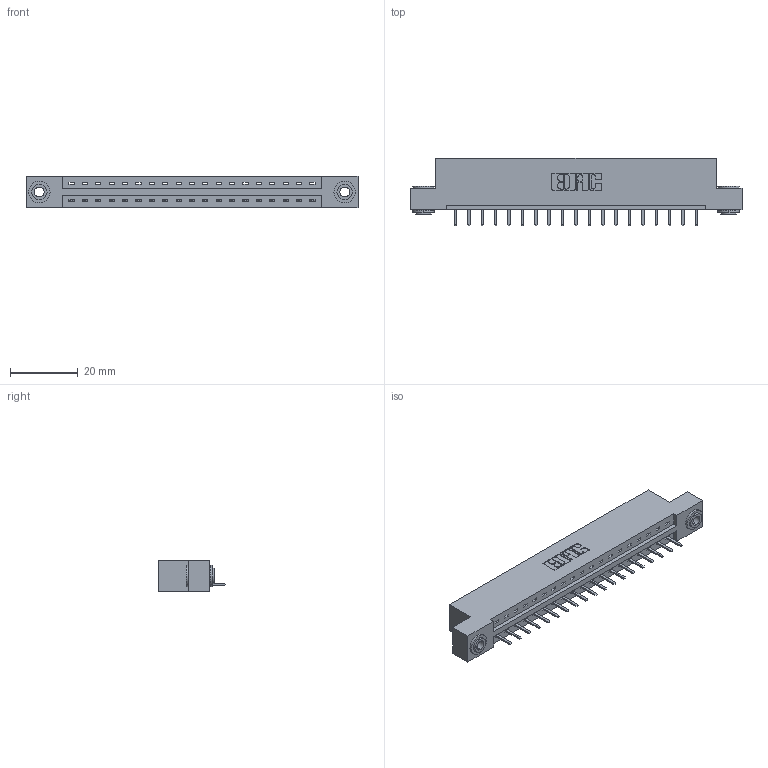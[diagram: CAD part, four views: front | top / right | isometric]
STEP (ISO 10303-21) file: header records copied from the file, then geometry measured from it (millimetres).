
FILE_DESCRIPTION (( 'STEP AP203' ), '1' );
FILE_NAME ('387-019-520-103.STEP', '2019-10-02T20:51:20', ( '' ), ( '' ), 'SwSTEP 2.0', 'SolidWorks 2016', '' );
FILE_SCHEMA (( 'CONFIG_CONTROL_DESIGN' ));
Length unit declared in the file: inch
Products named in the file (4): 337 Part_Flush Mounting Lugs - 0.156 Dia-TH; 387-019-520-103; 345-250-002_345-250-002-102; 345-292-001_345-293-120
Assembly tree (22 placements, depth 2):
  387-019-520-103
    337 Part_Flush Mounting Lugs - 0.156 Dia-TH
    345-292-001_345-293-120  x19
    345-250-002_345-250-002-102  x2
Bounding box: 98.3 x 20.02 x 9.4 mm (x, y, z)
Volume: 9893.3 mm3; surface area: 10131.6 mm2
Topology: 22 solids, 22 shells, 1406 faces, 4111 edges, 2686 vertices
Faces by surface type: plane 992, cylinder 406, cone 8
Entity records: 17862 total; most frequent: CARTESIAN_POINT 3098, ORIENTED_EDGE 3034, DIRECTION 2677, EDGE_CURVE 1517, VECTOR 1361, LINE 1361, VERTEX_POINT 1006, AXIS2_PLACEMENT_3D 658
